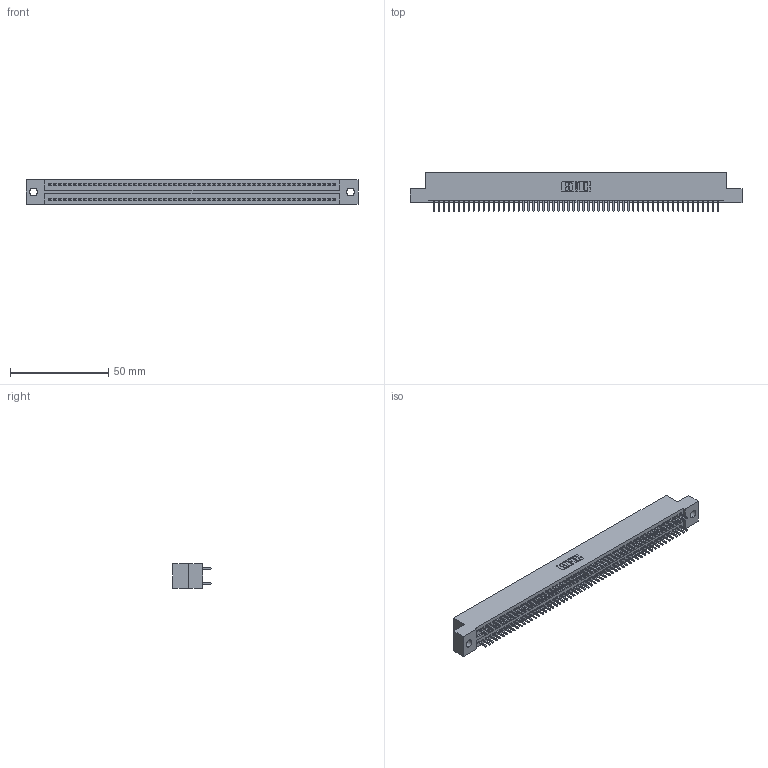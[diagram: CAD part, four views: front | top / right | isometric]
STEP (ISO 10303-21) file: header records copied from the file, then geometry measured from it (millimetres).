
FILE_DESCRIPTION (( 'STEP AP203' ), '1' );
FILE_NAME ('325-116-520-209.STEP', '2020-02-25T08:19:22', ( '' ), ( '' ), 'SwSTEP 2.0', 'SolidWorks 2016', '' );
FILE_SCHEMA (( 'CONFIG_CONTROL_DESIGN' ));
Length unit declared in the file: inch
Products named in the file (3): 325 Part_.160 TH; 325-116-520-209; 325-292-001_325-293-120
Assembly tree (117 placements, depth 2):
  325-116-520-209
    325 Part_.160 TH
    325-292-001_325-293-120  x116
Bounding box: 169.04 x 19.68 x 12.45 mm (x, y, z)
Volume: 21717.3 mm3; surface area: 26351.4 mm2
Topology: 117 solids, 117 shells, 6146 faces, 18291 edges, 12038 vertices
Faces by surface type: plane 4246, cylinder 1900
Entity records: 35265 total; most frequent: CARTESIAN_POINT 5826, ORIENTED_EDGE 5762, DIRECTION 4949, EDGE_CURVE 2881, VECTOR 2753, LINE 2753, VERTEX_POINT 1918, AXIS2_PLACEMENT_3D 1098
